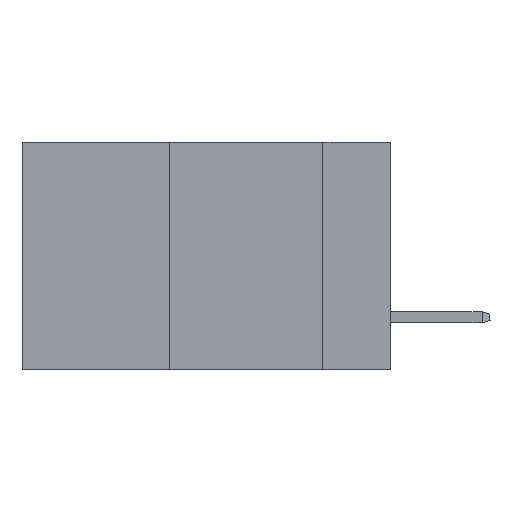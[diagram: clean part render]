
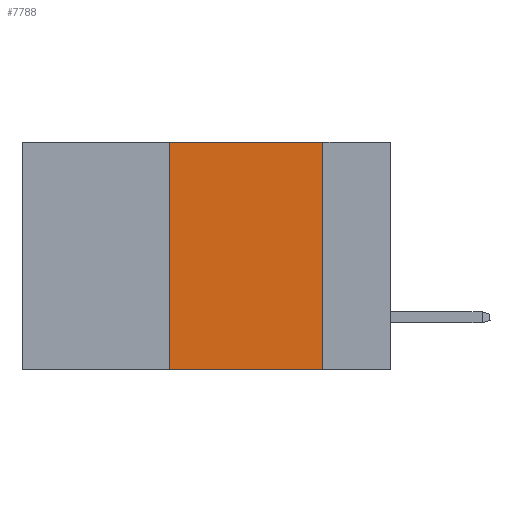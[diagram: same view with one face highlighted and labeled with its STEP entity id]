
A CAD part, left-side view. The second image highlights one B-rep face of the part: STEP entity #7788.
In plain terms, the highlighted planar face has unit normal (-1, 0, 0).
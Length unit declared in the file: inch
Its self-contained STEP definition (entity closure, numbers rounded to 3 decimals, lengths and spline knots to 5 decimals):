
#1379 = CARTESIAN_POINT ( 'NONE',  ( 0., 0.36, 0. ) ) ;
#5014 = ORIENTED_EDGE ( 'NONE', *, *, #18739, .T. ) ;
#5665 = VECTOR ( 'NONE', #25744, 39.37008 ) ;
#6899 = VERTEX_POINT ( 'NONE', #7998 ) ;
#7525 = LINE ( 'NONE', #41013, #36850 ) ;
#7788 = ADVANCED_FACE ( 'NONE', ( #10107 ), #19123, .F. ) ;
#7998 = CARTESIAN_POINT ( 'NONE',  ( 0., 0.36, 0. ) ) ;
#8937 = AXIS2_PLACEMENT_3D ( 'NONE', #36521, #15793, #30012 ) ;
#10107 = FACE_OUTER_BOUND ( 'NONE', #30631, .T. ) ;
#10161 = CARTESIAN_POINT ( 'NONE',  ( 0., 0.11, 0. ) ) ;
#10991 = VERTEX_POINT ( 'NONE', #36712 ) ;
#12797 = VERTEX_POINT ( 'NONE', #35506 ) ;
#13696 = VECTOR ( 'NONE', #14782, 39.37008 ) ;
#14782 = DIRECTION ( 'NONE',  ( 0., 0., -1. ) ) ;
#15420 = ORIENTED_EDGE ( 'NONE', *, *, #22675, .F. ) ;
#15793 = DIRECTION ( 'NONE',  ( 1., 0., 0. ) ) ;
#17558 = LINE ( 'NONE', #25831, #28332 ) ;
#18103 = LINE ( 'NONE', #1379, #5665 ) ;
#18739 = EDGE_CURVE ( 'NONE', #10991, #12797, #17558, .T. ) ;
#18983 = EDGE_CURVE ( 'NONE', #10991, #6899, #18103, .T. ) ;
#19123 = PLANE ( 'NONE',  #8937 ) ;
#22675 = EDGE_CURVE ( 'NONE', #6899, #27374, #7525, .T. ) ;
#25744 = DIRECTION ( 'NONE',  ( 0., 0., 1. ) ) ;
#25831 = CARTESIAN_POINT ( 'NONE',  ( 0., 0.6, -0.37 ) ) ;
#27374 = VERTEX_POINT ( 'NONE', #29028 ) ;
#28332 = VECTOR ( 'NONE', #31989, 39.37008 ) ;
#28557 = EDGE_CURVE ( 'NONE', #27374, #12797, #41790, .T. ) ;
#29028 = CARTESIAN_POINT ( 'NONE',  ( 0., 0.11, 0. ) ) ;
#30012 = DIRECTION ( 'NONE',  ( 0., 0., -1. ) ) ;
#30631 = EDGE_LOOP ( 'NONE', ( #37005, #15420, #39647, #5014 ) ) ;
#31989 = DIRECTION ( 'NONE',  ( 0., -1., 0. ) ) ;
#35506 = CARTESIAN_POINT ( 'NONE',  ( 0., 0.11, -0.37 ) ) ;
#36521 = CARTESIAN_POINT ( 'NONE',  ( 0., 0.6, 0. ) ) ;
#36712 = CARTESIAN_POINT ( 'NONE',  ( 0., 0.36, -0.37 ) ) ;
#36850 = VECTOR ( 'NONE', #40711, 39.37008 ) ;
#37005 = ORIENTED_EDGE ( 'NONE', *, *, #28557, .F. ) ;
#39647 = ORIENTED_EDGE ( 'NONE', *, *, #18983, .F. ) ;
#40711 = DIRECTION ( 'NONE',  ( 0., -1., 0. ) ) ;
#41013 = CARTESIAN_POINT ( 'NONE',  ( 0., 0.6, 0. ) ) ;
#41790 = LINE ( 'NONE', #10161, #13696 ) ;
